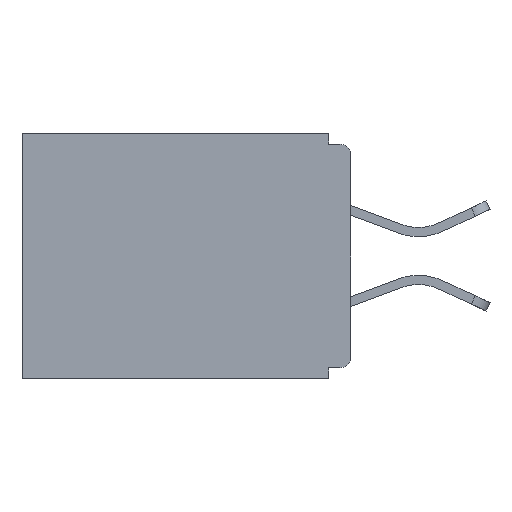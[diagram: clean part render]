
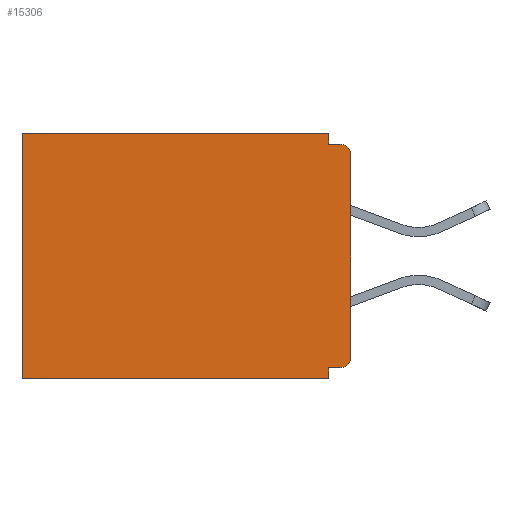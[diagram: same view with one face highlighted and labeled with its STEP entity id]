
A CAD part, left-side view. The second image highlights one B-rep face of the part: STEP entity #15306.
In plain terms, the highlighted planar face has unit normal (-1, 0, 0).
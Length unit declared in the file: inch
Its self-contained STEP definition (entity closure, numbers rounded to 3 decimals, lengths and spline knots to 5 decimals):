
#203 = LINE ( 'NONE', #14589, #25266 ) ;
#1040 = CARTESIAN_POINT ( 'NONE',  ( 0.298, 0., -0.313 ) ) ;
#1041 = FACE_OUTER_BOUND ( 'NONE', #11184, .T. ) ;
#1084 = DIRECTION ( 'NONE',  ( 0., 1., 0. ) ) ;
#1149 = CARTESIAN_POINT ( 'NONE',  ( 0.298, 0.015, -0.313 ) ) ;
#1379 = CARTESIAN_POINT ( 'NONE',  ( 0.298, 0., -0.015 ) ) ;
#3084 = DIRECTION ( 'NONE',  ( 1., 0., 0. ) ) ;
#3900 = VECTOR ( 'NONE', #17126, 39.37008 ) ;
#4068 = DIRECTION ( 'NONE',  ( 0., 1., 0. ) ) ;
#4252 = CARTESIAN_POINT ( 'NONE',  ( 0.298, 0., 0. ) ) ;
#6050 = CARTESIAN_POINT ( 'NONE',  ( 0.298, 0., 0. ) ) ;
#6067 = ORIENTED_EDGE ( 'NONE', *, *, #6937, .T. ) ;
#6937 = EDGE_CURVE ( 'NONE', #28981, #14872, #10555, .T. ) ;
#7504 = ORIENTED_EDGE ( 'NONE', *, *, #16184, .F. ) ;
#8173 = ORIENTED_EDGE ( 'NONE', *, *, #23235, .F. ) ;
#8214 = VECTOR ( 'NONE', #17983, 39.37008 ) ;
#8580 = DIRECTION ( 'NONE',  ( 0., 1., 0. ) ) ;
#9915 = ORIENTED_EDGE ( 'NONE', *, *, #21959, .F. ) ;
#10157 = DIRECTION ( 'NONE',  ( 0., 0., -1. ) ) ;
#10237 = EDGE_CURVE ( 'NONE', #14339, #20373, #14892, .T. ) ;
#10325 = EDGE_CURVE ( 'NONE', #29556, #25037, #15954, .T. ) ;
#10555 = CIRCLE ( 'NONE', #25860, 0.015 ) ;
#10574 = ORIENTED_EDGE ( 'NONE', *, *, #10325, .F. ) ;
#10581 = VECTOR ( 'NONE', #4068, 39.37008 ) ;
#11184 = EDGE_LOOP ( 'NONE', ( #23215, #8173, #9915, #16265, #24266, #10574, #7504, #15785, #6067, #15148 ) ) ;
#11304 = CARTESIAN_POINT ( 'NONE',  ( 0.298, 0.031, -0.328 ) ) ;
#11479 = VERTEX_POINT ( 'NONE', #11304 ) ;
#12400 = CARTESIAN_POINT ( 'NONE',  ( 0.298, 0., -0.03 ) ) ;
#13359 = CARTESIAN_POINT ( 'NONE',  ( 0.298, 0.015, -0.015 ) ) ;
#13435 = VECTOR ( 'NONE', #1084, 39.37008 ) ;
#13699 = EDGE_CURVE ( 'NONE', #23250, #25037, #203, .T. ) ;
#14282 = DIRECTION ( 'NONE',  ( 0., 0., -1. ) ) ;
#14339 = VERTEX_POINT ( 'NONE', #12400 ) ;
#14589 = CARTESIAN_POINT ( 'NONE',  ( 0.298, 0.46, 0. ) ) ;
#14845 = DIRECTION ( 'NONE',  ( -1., 0., 0. ) ) ;
#14872 = VERTEX_POINT ( 'NONE', #1040 ) ;
#14892 = CIRCLE ( 'NONE', #16946, 0.015 ) ;
#15148 = ORIENTED_EDGE ( 'NONE', *, *, #26966, .F. ) ;
#15306 = ADVANCED_FACE ( 'NONE', ( #1041 ), #26366, .F. ) ;
#15359 = CARTESIAN_POINT ( 'NONE',  ( 0.298, 0., -0.343 ) ) ;
#15566 = VERTEX_POINT ( 'NONE', #15834 ) ;
#15624 = CARTESIAN_POINT ( 'NONE',  ( 0.298, 0.46, 0. ) ) ;
#15785 = ORIENTED_EDGE ( 'NONE', *, *, #19803, .F. ) ;
#15834 = CARTESIAN_POINT ( 'NONE',  ( 0.298, 0.031, 0. ) ) ;
#15954 = LINE ( 'NONE', #15359, #13435 ) ;
#16184 = EDGE_CURVE ( 'NONE', #11479, #29556, #29315, .T. ) ;
#16265 = ORIENTED_EDGE ( 'NONE', *, *, #22152, .T. ) ;
#16916 = DIRECTION ( 'NONE',  ( 0., 0., -1. ) ) ;
#16938 = LINE ( 'NONE', #1379, #8214 ) ;
#16946 = AXIS2_PLACEMENT_3D ( 'NONE', #25862, #28083, #14282 ) ;
#17092 = CARTESIAN_POINT ( 'NONE',  ( 0.298, 0., 0. ) ) ;
#17126 = DIRECTION ( 'NONE',  ( 0., 0., -1. ) ) ;
#17983 = DIRECTION ( 'NONE',  ( 0., -1., 0. ) ) ;
#18845 = DIRECTION ( 'NONE',  ( 0., 0., -1. ) ) ;
#18852 = VECTOR ( 'NONE', #19274, 39.37008 ) ;
#19203 = LINE ( 'NONE', #19370, #3900 ) ;
#19274 = DIRECTION ( 'NONE',  ( 0., 0., -1. ) ) ;
#19370 = CARTESIAN_POINT ( 'NONE',  ( 0.298, 0.031, -0.343 ) ) ;
#19803 = EDGE_CURVE ( 'NONE', #28981, #11479, #23700, .T. ) ;
#20373 = VERTEX_POINT ( 'NONE', #13359 ) ;
#21833 = AXIS2_PLACEMENT_3D ( 'NONE', #17092, #3084, #23939 ) ;
#21959 = EDGE_CURVE ( 'NONE', #15566, #23474, #19203, .T. ) ;
#22152 = EDGE_CURVE ( 'NONE', #15566, #23250, #22455, .T. ) ;
#22455 = LINE ( 'NONE', #6050, #29385 ) ;
#23215 = ORIENTED_EDGE ( 'NONE', *, *, #10237, .T. ) ;
#23235 = EDGE_CURVE ( 'NONE', #23474, #20373, #16938, .T. ) ;
#23250 = VERTEX_POINT ( 'NONE', #15624 ) ;
#23474 = VERTEX_POINT ( 'NONE', #24506 ) ;
#23571 = CARTESIAN_POINT ( 'NONE',  ( 0.298, 0.031, -0.343 ) ) ;
#23700 = LINE ( 'NONE', #26965, #10581 ) ;
#23896 = CARTESIAN_POINT ( 'NONE',  ( 0.298, 0.015, -0.328 ) ) ;
#23939 = DIRECTION ( 'NONE',  ( 0., 0., -1. ) ) ;
#24266 = ORIENTED_EDGE ( 'NONE', *, *, #13699, .T. ) ;
#24506 = CARTESIAN_POINT ( 'NONE',  ( 0.298, 0.031, -0.015 ) ) ;
#25037 = VERTEX_POINT ( 'NONE', #28949 ) ;
#25266 = VECTOR ( 'NONE', #16916, 39.37008 ) ;
#25412 = LINE ( 'NONE', #4252, #18852 ) ;
#25860 = AXIS2_PLACEMENT_3D ( 'NONE', #1149, #14845, #10157 ) ;
#25862 = CARTESIAN_POINT ( 'NONE',  ( 0.298, 0.015, -0.03 ) ) ;
#26366 = PLANE ( 'NONE',  #21833 ) ;
#26420 = VECTOR ( 'NONE', #18845, 39.37008 ) ;
#26965 = CARTESIAN_POINT ( 'NONE',  ( 0.298, 0., -0.328 ) ) ;
#26966 = EDGE_CURVE ( 'NONE', #14339, #14872, #25412, .T. ) ;
#28083 = DIRECTION ( 'NONE',  ( -1., 0., 0. ) ) ;
#28949 = CARTESIAN_POINT ( 'NONE',  ( 0.298, 0.46, -0.343 ) ) ;
#28981 = VERTEX_POINT ( 'NONE', #23896 ) ;
#29315 = LINE ( 'NONE', #23571, #26420 ) ;
#29385 = VECTOR ( 'NONE', #8580, 39.37008 ) ;
#29556 = VERTEX_POINT ( 'NONE', #30042 ) ;
#30042 = CARTESIAN_POINT ( 'NONE',  ( 0.298, 0.031, -0.343 ) ) ;
